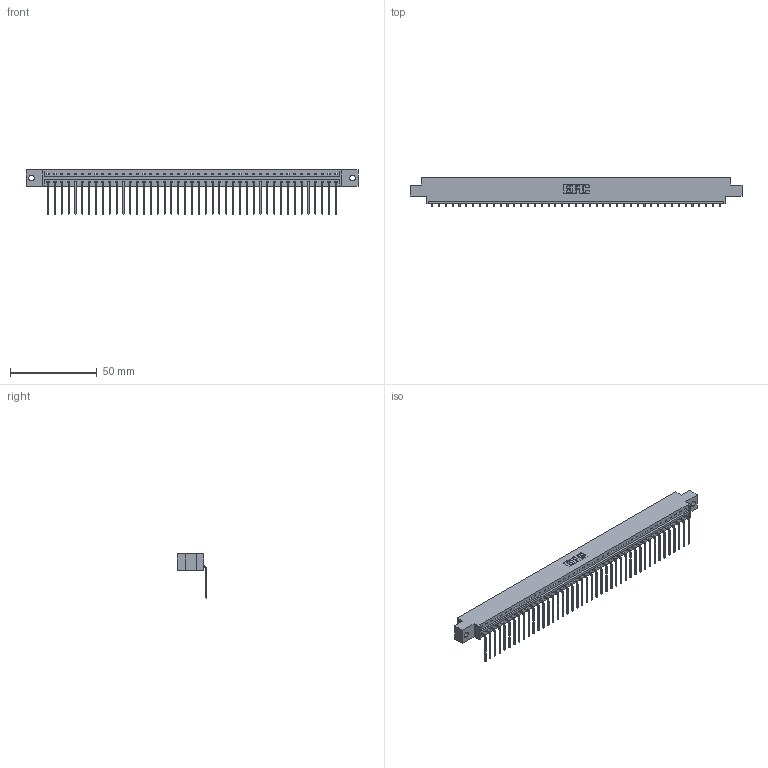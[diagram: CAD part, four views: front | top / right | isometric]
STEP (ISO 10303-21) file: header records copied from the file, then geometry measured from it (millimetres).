
FILE_DESCRIPTION (( 'STEP AP203' ), '1' );
FILE_NAME ('333-043-559-602.STEP', '2018-08-03T20:45:45', ( '' ), ( '' ), 'SwSTEP 2.0', 'SolidWorks 2016', '' );
FILE_SCHEMA (( 'CONFIG_CONTROL_DESIGN' ));
Length unit declared in the file: inch
Products named in the file (3): 333 Part_Offset - .128 Dia; 345-292-001_558 559 Tail - 1; 333-043-559-602
Assembly tree (44 placements, depth 2):
  333-043-559-602
    333 Part_Offset - .128 Dia
    345-292-001_558 559 Tail - 1  x43
Bounding box: 191.92 x 17.09 x 25.53 mm (x, y, z)
Volume: 19200.2 mm3; surface area: 21585.1 mm2
Topology: 44 solids, 44 shells, 2698 faces, 8149 edges, 5374 vertices
Faces by surface type: plane 1966, cylinder 732
Entity records: 26377 total; most frequent: CARTESIAN_POINT 4559, ORIENTED_EDGE 4538, DIRECTION 3843, EDGE_CURVE 2269, VECTOR 2141, LINE 2141, VERTEX_POINT 1510, AXIS2_PLACEMENT_3D 851
